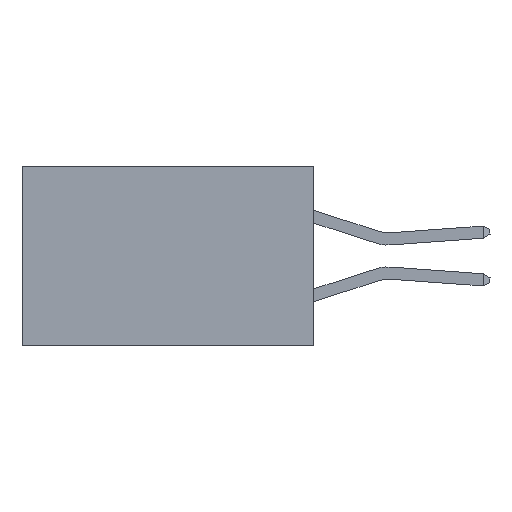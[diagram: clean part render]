
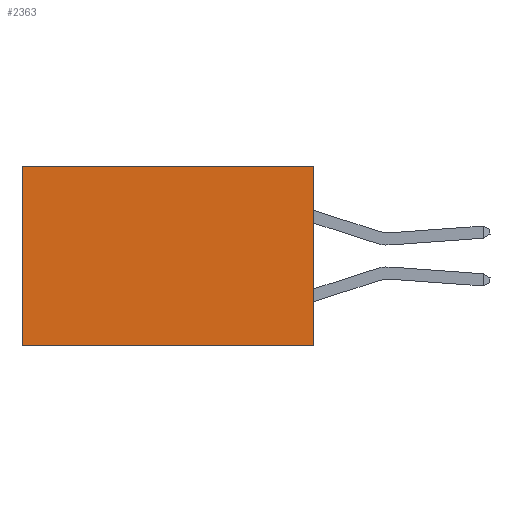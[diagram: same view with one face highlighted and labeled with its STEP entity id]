
A CAD part, left-side view. The second image highlights one B-rep face of the part: STEP entity #2363.
In plain terms, the highlighted planar face has unit normal (-1, 0, 0).
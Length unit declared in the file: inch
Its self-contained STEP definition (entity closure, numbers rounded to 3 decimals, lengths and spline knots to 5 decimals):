
#792 = FACE_OUTER_BOUND ( 'NONE', #14257, .T. ) ;
#1367 = EDGE_CURVE ( 'NONE', #18661, #3603, #8964, .T. ) ;
#2073 = VECTOR ( 'NONE', #17563, 39.37008 ) ;
#2363 = ADVANCED_FACE ( 'NONE', ( #792 ), #28167, .F. ) ;
#2984 = EDGE_CURVE ( 'NONE', #22203, #3603, #17891, .T. ) ;
#3603 = VERTEX_POINT ( 'NONE', #16694 ) ;
#3895 = DIRECTION ( 'NONE',  ( 1., 0., 0. ) ) ;
#5876 = LINE ( 'NONE', #17290, #25989 ) ;
#5936 = CARTESIAN_POINT ( 'NONE',  ( 0.2875, 0., -0.37 ) ) ;
#7462 = VECTOR ( 'NONE', #27181, 39.37008 ) ;
#8964 = LINE ( 'NONE', #10379, #22911 ) ;
#9625 = VERTEX_POINT ( 'NONE', #27574 ) ;
#10379 = CARTESIAN_POINT ( 'NONE',  ( 0.2875, 0.6, 0. ) ) ;
#11478 = CARTESIAN_POINT ( 'NONE',  ( 0.2875, 0., 0. ) ) ;
#12049 = DIRECTION ( 'NONE',  ( 0., 0., -1. ) ) ;
#12950 = EDGE_CURVE ( 'NONE', #9625, #18661, #14513, .T. ) ;
#14257 = EDGE_LOOP ( 'NONE', ( #25799, #32507, #25626, #19099 ) ) ;
#14513 = LINE ( 'NONE', #11478, #7462 ) ;
#15923 = AXIS2_PLACEMENT_3D ( 'NONE', #32124, #3895, #30100 ) ;
#16694 = CARTESIAN_POINT ( 'NONE',  ( 0.2875, 0.6, -0.37 ) ) ;
#17290 = CARTESIAN_POINT ( 'NONE',  ( 0.2875, 0., 0. ) ) ;
#17563 = DIRECTION ( 'NONE',  ( 0., 1., 0. ) ) ;
#17891 = LINE ( 'NONE', #25060, #2073 ) ;
#18661 = VERTEX_POINT ( 'NONE', #21766 ) ;
#19099 = ORIENTED_EDGE ( 'NONE', *, *, #12950, .T. ) ;
#21695 = EDGE_CURVE ( 'NONE', #9625, #22203, #5876, .T. ) ;
#21766 = CARTESIAN_POINT ( 'NONE',  ( 0.2875, 0.6, 0. ) ) ;
#22203 = VERTEX_POINT ( 'NONE', #5936 ) ;
#22911 = VECTOR ( 'NONE', #33759, 39.37008 ) ;
#25060 = CARTESIAN_POINT ( 'NONE',  ( 0.2875, 0., -0.37 ) ) ;
#25626 = ORIENTED_EDGE ( 'NONE', *, *, #21695, .F. ) ;
#25799 = ORIENTED_EDGE ( 'NONE', *, *, #1367, .T. ) ;
#25989 = VECTOR ( 'NONE', #12049, 39.37008 ) ;
#27181 = DIRECTION ( 'NONE',  ( 0., 1., 0. ) ) ;
#27574 = CARTESIAN_POINT ( 'NONE',  ( 0.2875, 0., 0. ) ) ;
#28167 = PLANE ( 'NONE',  #15923 ) ;
#30100 = DIRECTION ( 'NONE',  ( 0., 0., -1. ) ) ;
#32124 = CARTESIAN_POINT ( 'NONE',  ( 0.2875, 0., 0. ) ) ;
#32507 = ORIENTED_EDGE ( 'NONE', *, *, #2984, .F. ) ;
#33759 = DIRECTION ( 'NONE',  ( 0., 0., -1. ) ) ;
